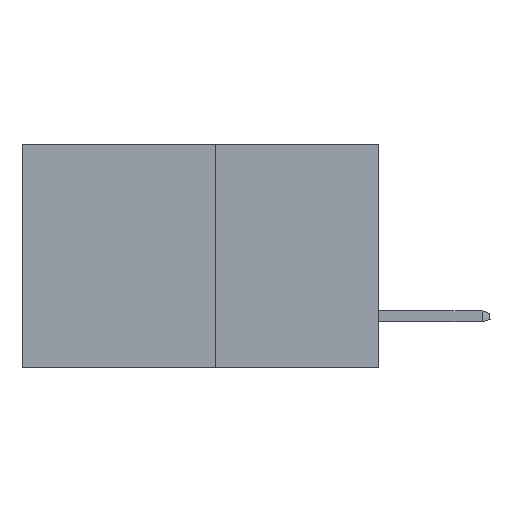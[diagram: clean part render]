
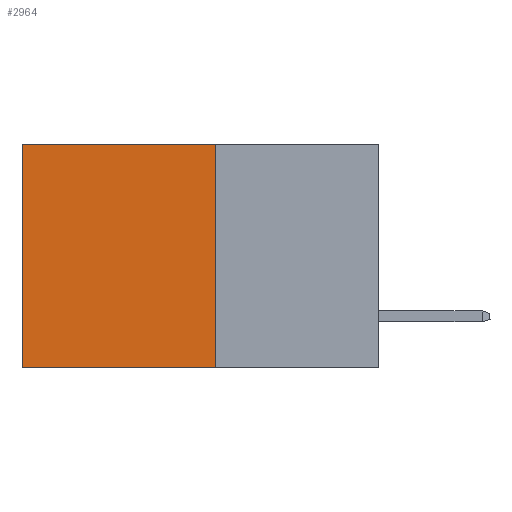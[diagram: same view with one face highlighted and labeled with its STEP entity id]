
A CAD part, left-side view. The second image highlights one B-rep face of the part: STEP entity #2964.
In plain terms, the highlighted planar face has unit normal (-1, 0, 0).
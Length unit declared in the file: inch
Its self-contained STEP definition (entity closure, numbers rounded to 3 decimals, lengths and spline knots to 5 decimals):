
#199 = CARTESIAN_POINT ( 'NONE',  ( 0.277, 0.59, -0.37 ) ) ;
#489 = PLANE ( 'NONE',  #6663 ) ;
#1591 = CARTESIAN_POINT ( 'NONE',  ( 0.277, 0.27, -0.37 ) ) ;
#1900 = EDGE_CURVE ( 'NONE', #6231, #10459, #9227, .T. ) ;
#2176 = VECTOR ( 'NONE', #6502, 39.37008 ) ;
#2502 = EDGE_CURVE ( 'NONE', #4153, #7672, #7588, .T. ) ;
#2757 = EDGE_CURVE ( 'NONE', #10459, #7672, #9203, .T. ) ;
#2964 = ADVANCED_FACE ( 'NONE', ( #9604 ), #489, .F. ) ;
#3663 = CARTESIAN_POINT ( 'NONE',  ( 0.277, 0.27, 0. ) ) ;
#4144 = VECTOR ( 'NONE', #4572, 39.37008 ) ;
#4153 = VERTEX_POINT ( 'NONE', #11429 ) ;
#4461 = CARTESIAN_POINT ( 'NONE',  ( 0.277, 0.27, 0. ) ) ;
#4572 = DIRECTION ( 'NONE',  ( 0., 1., 0. ) ) ;
#5114 = VECTOR ( 'NONE', #9849, 39.37008 ) ;
#5444 = ORIENTED_EDGE ( 'NONE', *, *, #2757, .F. ) ;
#6042 = DIRECTION ( 'NONE',  ( 1., 0., 0. ) ) ;
#6231 = VERTEX_POINT ( 'NONE', #4461 ) ;
#6431 = CARTESIAN_POINT ( 'NONE',  ( 0.277, 0.27, -0.37 ) ) ;
#6502 = DIRECTION ( 'NONE',  ( 0., 1., 0. ) ) ;
#6663 = AXIS2_PLACEMENT_3D ( 'NONE', #6431, #6042, #8564 ) ;
#6892 = ORIENTED_EDGE ( 'NONE', *, *, #6995, .T. ) ;
#6995 = EDGE_CURVE ( 'NONE', #6231, #4153, #8707, .T. ) ;
#7318 = DIRECTION ( 'NONE',  ( 0., 0., -1. ) ) ;
#7474 = CARTESIAN_POINT ( 'NONE',  ( 0.277, 0.27, -0.37 ) ) ;
#7588 = LINE ( 'NONE', #9648, #5114 ) ;
#7672 = VERTEX_POINT ( 'NONE', #199 ) ;
#8350 = CARTESIAN_POINT ( 'NONE',  ( 0.277, 0.27, -0.37 ) ) ;
#8564 = DIRECTION ( 'NONE',  ( 0., 0., -1. ) ) ;
#8707 = LINE ( 'NONE', #3663, #4144 ) ;
#8943 = VECTOR ( 'NONE', #7318, 39.37008 ) ;
#9203 = LINE ( 'NONE', #7474, #2176 ) ;
#9227 = LINE ( 'NONE', #1591, #8943 ) ;
#9396 = EDGE_LOOP ( 'NONE', ( #11693, #5444, #10731, #6892 ) ) ;
#9604 = FACE_OUTER_BOUND ( 'NONE', #9396, .T. ) ;
#9648 = CARTESIAN_POINT ( 'NONE',  ( 0.277, 0.59, -0.37 ) ) ;
#9849 = DIRECTION ( 'NONE',  ( 0., 0., -1. ) ) ;
#10459 = VERTEX_POINT ( 'NONE', #8350 ) ;
#10731 = ORIENTED_EDGE ( 'NONE', *, *, #1900, .F. ) ;
#11429 = CARTESIAN_POINT ( 'NONE',  ( 0.277, 0.59, 0. ) ) ;
#11693 = ORIENTED_EDGE ( 'NONE', *, *, #2502, .T. ) ;
